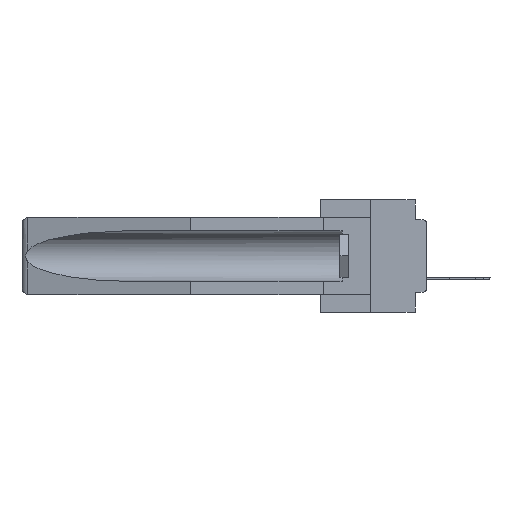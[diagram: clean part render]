
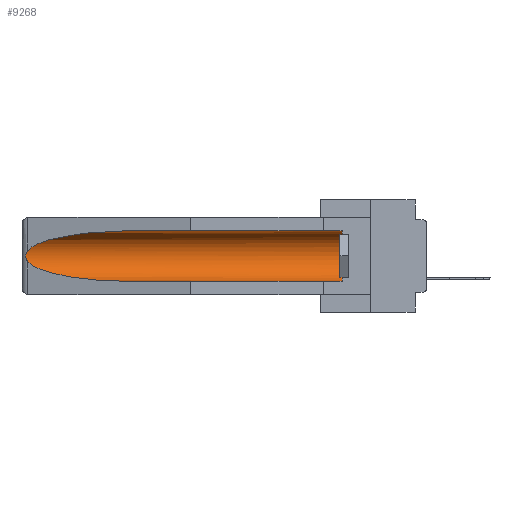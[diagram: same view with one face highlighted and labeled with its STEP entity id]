
A CAD part, left-side view. The second image highlights one B-rep face of the part: STEP entity #9268.
In plain terms, the highlighted cylindrical face has radius 2.857 mm (diameter 5.715 mm), a partial arc.
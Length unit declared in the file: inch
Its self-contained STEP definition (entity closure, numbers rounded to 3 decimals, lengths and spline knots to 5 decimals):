
#774 = VECTOR ( 'NONE', #2182, 39.37008 ) ;
#2104 = VERTEX_POINT ( 'NONE', #26001 ) ;
#2182 = DIRECTION ( 'NONE',  ( 0., 1., 0. ) ) ;
#2780 = CARTESIAN_POINT ( 'NONE',  ( 0.155, 0.126, -0.059 ) ) ;
#3018 = ORIENTED_EDGE ( 'NONE', *, *, #26862, .F. ) ;
#3440 = CARTESIAN_POINT ( 'NONE',  ( 0.155, 1.07973, -0.284 ) ) ;
#3501 = CARTESIAN_POINT ( 'NONE',  ( 0.26597, 1.5296, -0.19026 ) ) ;
#4843 = ORIENTED_EDGE ( 'NONE', *, *, #6217, .T. ) ;
#4859 = LINE ( 'NONE', #26186, #21683 ) ;
#5372 = DIRECTION ( 'NONE',  ( 0., 1., 0. ) ) ;
#5961 = ORIENTED_EDGE ( 'NONE', *, *, #20108, .T. ) ;
#6082 = CYLINDRICAL_SURFACE ( 'NONE', #30491, 0.1125 ) ;
#6217 = EDGE_CURVE ( 'NONE', #2104, #32985, #10402, .T. ) ;
#6617 = CARTESIAN_POINT ( 'NONE',  ( 0.26537, 1.52718, -0.19328 ) ) ;
#6812 = CARTESIAN_POINT ( 'NONE',  ( 0.155, 1.07973, -0.059 ) ) ;
#6978 = CARTESIAN_POINT ( 'NONE',  ( 0.25451, 1.48313, -0.24835 ) ) ;
#7492 = VERTEX_POINT ( 'NONE', #2780 ) ;
#9135 = ORIENTED_EDGE ( 'NONE', *, *, #15701, .T. ) ;
#9268 = ADVANCED_FACE ( 'NONE', ( #21715 ), #6082, .F. ) ;
#9519 = EDGE_CURVE ( 'NONE', #7492, #26667, #4859, .T. ) ;
#10402 =( BOUNDED_CURVE ( )  B_SPLINE_CURVE ( 3, ( #6617, #6978, #33890, #3440 ),
 .UNSPECIFIED., .F., .F. ) 
 B_SPLINE_CURVE_WITH_KNOTS ( ( 4, 4 ),
 ( 0.1948, 1.5708 ),
 .UNSPECIFIED. ) 
 CURVE ( )  GEOMETRIC_REPRESENTATION_ITEM ( )  RATIONAL_B_SPLINE_CURVE ( ( 1., 0.848, 0.848, 1. ) ) 
 REPRESENTATION_ITEM ( '' )  );
#10512 = CARTESIAN_POINT ( 'NONE',  ( 0.26537, 1.52718, -0.14972 ) ) ;
#10734 = CARTESIAN_POINT ( 'NONE',  ( 0.2673, 1.5327, -0.16383 ) ) ;
#11132 = CARTESIAN_POINT ( 'NONE',  ( 0.155, 1.07973, -0.059 ) ) ;
#11186 = DIRECTION ( 'NONE',  ( 0., 0., 1. ) ) ;
#11903 = CARTESIAN_POINT ( 'NONE',  ( 0.2675, 1.53308, -0.17534 ) ) ;
#12355 = ORIENTED_EDGE ( 'NONE', *, *, #18845, .T. ) ;
#12471 = CARTESIAN_POINT ( 'NONE',  ( 0.155, 0.126, -0.284 ) ) ;
#13770 = CARTESIAN_POINT ( 'NONE',  ( 0.26537, 1.52718, -0.14972 ) ) ;
#14020 = B_SPLINE_CURVE_WITH_KNOTS ( 'NONE', 3,
 ( #10512, #28915, #26390, #10734, #17063, #11903, #16585, #19242, #3501, #27286 ),
 .UNSPECIFIED., .F., .F.,
 ( 4, 2, 2, 2, 4 ),
 ( 0., 0.00029, 0.00058, 0.00087, 0.00117 ),
 .UNSPECIFIED. ) ;
#14279 = CARTESIAN_POINT ( 'NONE',  ( 0.26537, 1.52718, -0.14972 ) ) ;
#14605 = DIRECTION ( 'NONE',  ( 0., 0., 1. ) ) ;
#15701 = EDGE_CURVE ( 'NONE', #29963, #7492, #25508, .T. ) ;
#16585 = CARTESIAN_POINT ( 'NONE',  ( 0.2673, 1.53269, -0.17917 ) ) ;
#17063 = CARTESIAN_POINT ( 'NONE',  ( 0.2675, 1.53308, -0.16763 ) ) ;
#17882 = VERTEX_POINT ( 'NONE', #13770 ) ;
#18845 = EDGE_CURVE ( 'NONE', #17882, #2104, #14020, .T. ) ;
#18969 = AXIS2_PLACEMENT_3D ( 'NONE', #26713, #26938, #11186 ) ;
#19242 = CARTESIAN_POINT ( 'NONE',  ( 0.26655, 1.53094, -0.18657 ) ) ;
#20108 = EDGE_CURVE ( 'NONE', #26667, #17882, #27685, .T. ) ;
#21683 = VECTOR ( 'NONE', #5372, 39.37008 ) ;
#21715 = FACE_OUTER_BOUND ( 'NONE', #28057, .T. ) ;
#23822 = ORIENTED_EDGE ( 'NONE', *, *, #9519, .T. ) ;
#24003 = CARTESIAN_POINT ( 'NONE',  ( 0.155, 1.07973, -0.284 ) ) ;
#25067 = CARTESIAN_POINT ( 'NONE',  ( 0.155, -0.30754, -0.1715 ) ) ;
#25068 = CARTESIAN_POINT ( 'NONE',  ( 0.155, -0.30754, -0.284 ) ) ;
#25229 = CARTESIAN_POINT ( 'NONE',  ( 0.21114, 1.30732, -0.059 ) ) ;
#25508 = CIRCLE ( 'NONE', #18969, 0.1125 ) ;
#26001 = CARTESIAN_POINT ( 'NONE',  ( 0.26537, 1.52718, -0.19328 ) ) ;
#26186 = CARTESIAN_POINT ( 'NONE',  ( 0.155, -0.30754, -0.059 ) ) ;
#26390 = CARTESIAN_POINT ( 'NONE',  ( 0.26654, 1.53092, -0.15636 ) ) ;
#26667 = VERTEX_POINT ( 'NONE', #11132 ) ;
#26713 = CARTESIAN_POINT ( 'NONE',  ( 0.155, 0.126, -0.1715 ) ) ;
#26862 = EDGE_CURVE ( 'NONE', #29963, #32985, #32863, .T. ) ;
#26938 = DIRECTION ( 'NONE',  ( 0., -1., 0. ) ) ;
#27286 = CARTESIAN_POINT ( 'NONE',  ( 0.26537, 1.52718, -0.19328 ) ) ;
#27685 =( BOUNDED_CURVE ( )  B_SPLINE_CURVE ( 3, ( #6812, #25229, #30006, #14279 ),
 .UNSPECIFIED., .F., .F. ) 
 B_SPLINE_CURVE_WITH_KNOTS ( ( 4, 4 ),
 ( 4.71239, 6.08839 ),
 .UNSPECIFIED. ) 
 CURVE ( )  GEOMETRIC_REPRESENTATION_ITEM ( )  RATIONAL_B_SPLINE_CURVE ( ( 1., 0.848, 0.848, 1. ) ) 
 REPRESENTATION_ITEM ( '' )  );
#28057 = EDGE_LOOP ( 'NONE', ( #5961, #12355, #4843, #3018, #9135, #23822 ) ) ;
#28915 = CARTESIAN_POINT ( 'NONE',  ( 0.26597, 1.52961, -0.15275 ) ) ;
#29963 = VERTEX_POINT ( 'NONE', #12471 ) ;
#30006 = CARTESIAN_POINT ( 'NONE',  ( 0.25451, 1.48313, -0.09465 ) ) ;
#30491 = AXIS2_PLACEMENT_3D ( 'NONE', #25067, #33453, #14605 ) ;
#32863 = LINE ( 'NONE', #25068, #774 ) ;
#32985 = VERTEX_POINT ( 'NONE', #24003 ) ;
#33453 = DIRECTION ( 'NONE',  ( 0., 1., 0. ) ) ;
#33890 = CARTESIAN_POINT ( 'NONE',  ( 0.21114, 1.30732, -0.284 ) ) ;
